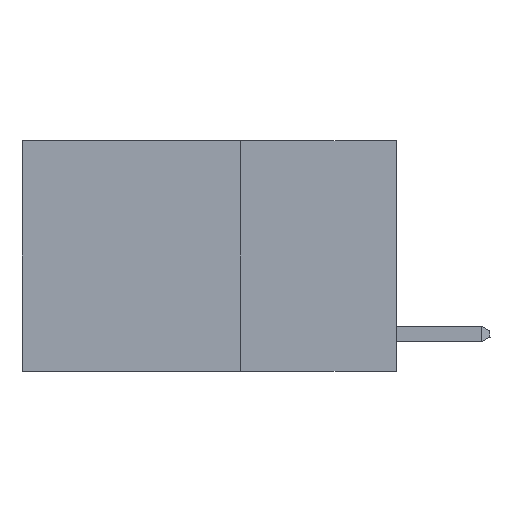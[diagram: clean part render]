
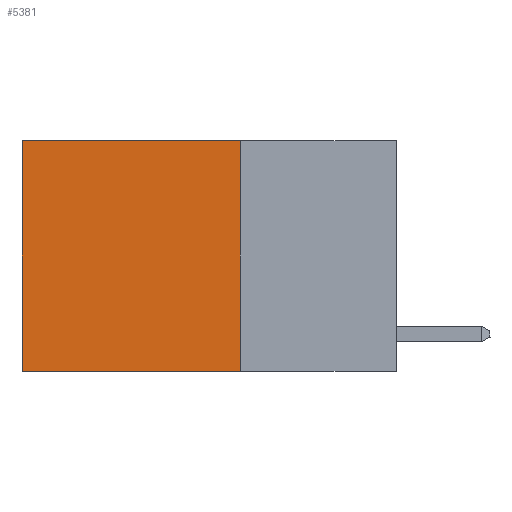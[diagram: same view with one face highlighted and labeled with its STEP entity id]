
A CAD part, left-side view. The second image highlights one B-rep face of the part: STEP entity #5381.
In plain terms, the highlighted planar face has unit normal (-1, 0, 0).
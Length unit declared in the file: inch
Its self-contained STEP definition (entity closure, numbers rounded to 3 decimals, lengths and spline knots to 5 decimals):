
#308 = AXIS2_PLACEMENT_3D ( 'NONE', #8404, #3908, #14392 ) ;
#312 = ORIENTED_EDGE ( 'NONE', *, *, #10114, .T. ) ;
#354 = LINE ( 'NONE', #6502, #7918 ) ;
#997 = DIRECTION ( 'NONE',  ( 0., 1., 0. ) ) ;
#1302 = VECTOR ( 'NONE', #18190, 39.37008 ) ;
#3096 = LINE ( 'NONE', #10034, #14112 ) ;
#3236 = FACE_OUTER_BOUND ( 'NONE', #5028, .T. ) ;
#3755 = VERTEX_POINT ( 'NONE', #11975 ) ;
#3908 = DIRECTION ( 'NONE',  ( 1., 0., 0. ) ) ;
#4355 = ORIENTED_EDGE ( 'NONE', *, *, #10168, .F. ) ;
#4936 = CARTESIAN_POINT ( 'NONE',  ( 0.2625, 0.6, 0. ) ) ;
#5028 = EDGE_LOOP ( 'NONE', ( #13934, #5988, #4355, #312 ) ) ;
#5381 = ADVANCED_FACE ( 'NONE', ( #3236 ), #12905, .F. ) ;
#5988 = ORIENTED_EDGE ( 'NONE', *, *, #18582, .F. ) ;
#6144 = VECTOR ( 'NONE', #7978, 39.37008 ) ;
#6502 = CARTESIAN_POINT ( 'NONE',  ( 0.2625, 0.25, 0. ) ) ;
#7380 = VERTEX_POINT ( 'NONE', #18282 ) ;
#7918 = VECTOR ( 'NONE', #15424, 39.37008 ) ;
#7978 = DIRECTION ( 'NONE',  ( 0., 0., -1. ) ) ;
#8404 = CARTESIAN_POINT ( 'NONE',  ( 0.2625, 0.25, 0. ) ) ;
#9018 = VERTEX_POINT ( 'NONE', #14248 ) ;
#9329 = LINE ( 'NONE', #13826, #1302 ) ;
#10034 = CARTESIAN_POINT ( 'NONE',  ( 0.2625, 0.25, -0.37 ) ) ;
#10114 = EDGE_CURVE ( 'NONE', #7380, #9018, #9329, .T. ) ;
#10168 = EDGE_CURVE ( 'NONE', #7380, #10221, #354, .T. ) ;
#10221 = VERTEX_POINT ( 'NONE', #14008 ) ;
#11975 = CARTESIAN_POINT ( 'NONE',  ( 0.2625, 0.6, -0.37 ) ) ;
#12905 = PLANE ( 'NONE',  #308 ) ;
#13826 = CARTESIAN_POINT ( 'NONE',  ( 0.2625, 0.25, 0. ) ) ;
#13934 = ORIENTED_EDGE ( 'NONE', *, *, #19001, .T. ) ;
#14008 = CARTESIAN_POINT ( 'NONE',  ( 0.2625, 0.25, -0.37 ) ) ;
#14112 = VECTOR ( 'NONE', #997, 39.37008 ) ;
#14248 = CARTESIAN_POINT ( 'NONE',  ( 0.2625, 0.6, 0. ) ) ;
#14392 = DIRECTION ( 'NONE',  ( 0., 0., -1. ) ) ;
#15424 = DIRECTION ( 'NONE',  ( 0., 0., -1. ) ) ;
#17945 = LINE ( 'NONE', #4936, #6144 ) ;
#18190 = DIRECTION ( 'NONE',  ( 0., 1., 0. ) ) ;
#18282 = CARTESIAN_POINT ( 'NONE',  ( 0.2625, 0.25, 0. ) ) ;
#18582 = EDGE_CURVE ( 'NONE', #10221, #3755, #3096, .T. ) ;
#19001 = EDGE_CURVE ( 'NONE', #9018, #3755, #17945, .T. ) ;
